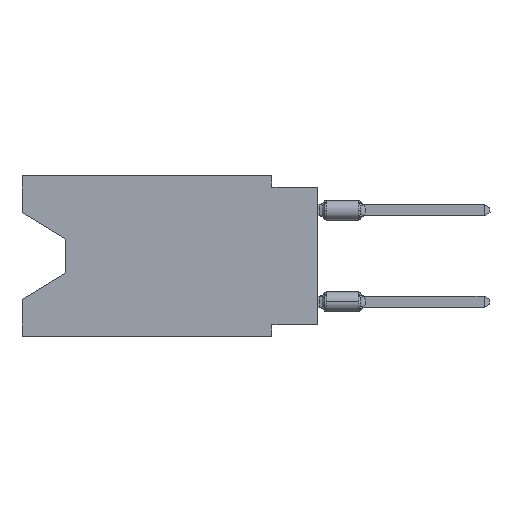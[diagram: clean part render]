
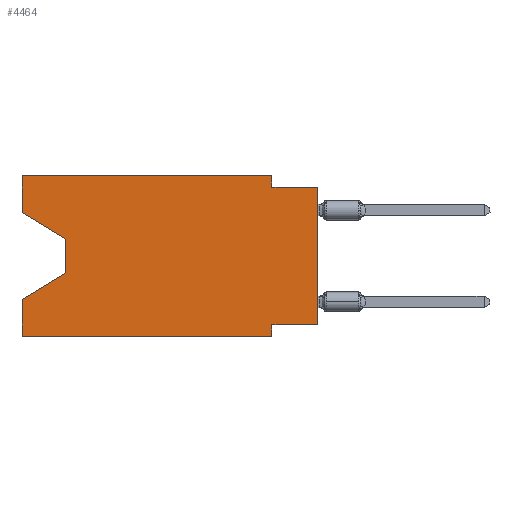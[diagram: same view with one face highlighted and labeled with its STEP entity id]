
A CAD part, left-side view. The second image highlights one B-rep face of the part: STEP entity #4464.
In plain terms, the highlighted planar face has unit normal (-1, 0, 0).
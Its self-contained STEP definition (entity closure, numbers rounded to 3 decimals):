
#127 = EDGE_CURVE ( 'NONE', #20466, #29470, #26719, .T. ) ;
#238 = DIRECTION ( 'NONE',  ( 0., 0., -1. ) ) ;
#277 = CARTESIAN_POINT ( 'NONE',  ( 0., 16.383, -2.038 ) ) ;
#307 = VERTEX_POINT ( 'NONE', #22963 ) ;
#825 = DIRECTION ( 'NONE',  ( 0., 0.855, -0.519 ) ) ;
#912 = VECTOR ( 'NONE', #4935, 1000. ) ;
#986 = CARTESIAN_POINT ( 'NONE',  ( 0., 13.97, -5.385 ) ) ;
#1016 = VERTEX_POINT ( 'NONE', #8411 ) ;
#1348 = VERTEX_POINT ( 'NONE', #986 ) ;
#1746 = EDGE_CURVE ( 'NONE', #307, #1348, #17062, .T. ) ;
#1863 = VECTOR ( 'NONE', #26538, 1000. ) ;
#1892 = DIRECTION ( 'NONE',  ( 0., -0.855, -0.519 ) ) ;
#2112 = CARTESIAN_POINT ( 'NONE',  ( 0., 0., -0.635 ) ) ;
#2147 = CARTESIAN_POINT ( 'NONE',  ( 0., 0., 0. ) ) ;
#2938 = VECTOR ( 'NONE', #26191, 1000. ) ;
#3699 = CARTESIAN_POINT ( 'NONE',  ( 0., 16.383, 0. ) ) ;
#3828 = VECTOR ( 'NONE', #28101, 1000. ) ;
#4464 = ADVANCED_FACE ( 'NONE', ( #6754 ), #16173, .F. ) ;
#4853 = LINE ( 'NONE', #12259, #29091 ) ;
#4935 = DIRECTION ( 'NONE',  ( 0., 1., 0. ) ) ;
#5178 = EDGE_CURVE ( 'NONE', #7450, #18401, #17626, .T. ) ;
#5221 = VERTEX_POINT ( 'NONE', #19931 ) ;
#5385 = VECTOR ( 'NONE', #11544, 1000. ) ;
#5508 = CARTESIAN_POINT ( 'NONE',  ( 0., 0., -8.255 ) ) ;
#6181 = CARTESIAN_POINT ( 'NONE',  ( 0., 2.54, -0.635 ) ) ;
#6455 = CARTESIAN_POINT ( 'NONE',  ( 0., 16.383, 0. ) ) ;
#6513 = CARTESIAN_POINT ( 'NONE',  ( 0., 16.383, -2.038 ) ) ;
#6754 = FACE_OUTER_BOUND ( 'NONE', #8732, .T. ) ;
#6927 = VERTEX_POINT ( 'NONE', #28974 ) ;
#7450 = VERTEX_POINT ( 'NONE', #6181 ) ;
#7916 = LINE ( 'NONE', #12678, #8224 ) ;
#8224 = VECTOR ( 'NONE', #825, 1000. ) ;
#8411 = CARTESIAN_POINT ( 'NONE',  ( 0., 2.54, -8.255 ) ) ;
#8651 = ORIENTED_EDGE ( 'NONE', *, *, #22971, .F. ) ;
#8732 = EDGE_LOOP ( 'NONE', ( #28680, #16036, #20191, #23287, #11457, #8651, #28444, #9402, #25509, #11028, #11565, #10864 ) ) ;
#9210 = DIRECTION ( 'NONE',  ( 1., 0., 0. ) ) ;
#9402 = ORIENTED_EDGE ( 'NONE', *, *, #22420, .T. ) ;
#9541 = LINE ( 'NONE', #28402, #912 ) ;
#9698 = CARTESIAN_POINT ( 'NONE',  ( 0., 16.383, 0. ) ) ;
#9869 = LINE ( 'NONE', #19272, #25025 ) ;
#10098 = DIRECTION ( 'NONE',  ( 0., 0., -1. ) ) ;
#10293 = VERTEX_POINT ( 'NONE', #5508 ) ;
#10674 = EDGE_CURVE ( 'NONE', #29470, #7450, #4853, .T. ) ;
#10826 = CARTESIAN_POINT ( 'NONE',  ( 0., 0., -0.635 ) ) ;
#10864 = ORIENTED_EDGE ( 'NONE', *, *, #19400, .F. ) ;
#11028 = ORIENTED_EDGE ( 'NONE', *, *, #10674, .F. ) ;
#11457 = ORIENTED_EDGE ( 'NONE', *, *, #25524, .T. ) ;
#11544 = DIRECTION ( 'NONE',  ( 0., 0., 1. ) ) ;
#11565 = ORIENTED_EDGE ( 'NONE', *, *, #127, .F. ) ;
#12259 = CARTESIAN_POINT ( 'NONE',  ( 0., 2.54, 0. ) ) ;
#12345 = DIRECTION ( 'NONE',  ( 0., -1., 0. ) ) ;
#12559 = VECTOR ( 'NONE', #24381, 1000. ) ;
#12678 = CARTESIAN_POINT ( 'NONE',  ( 0., 13.97, -5.385 ) ) ;
#14000 = DIRECTION ( 'NONE',  ( 0., 0., -1. ) ) ;
#14806 = LINE ( 'NONE', #9698, #1863 ) ;
#16036 = ORIENTED_EDGE ( 'NONE', *, *, #1746, .T. ) ;
#16079 = CARTESIAN_POINT ( 'NONE',  ( 0., 16.383, 0. ) ) ;
#16173 = PLANE ( 'NONE',  #30068 ) ;
#16773 = CARTESIAN_POINT ( 'NONE',  ( 0., 16.383, -6.852 ) ) ;
#17062 = LINE ( 'NONE', #21830, #27928 ) ;
#17350 = EDGE_CURVE ( 'NONE', #19780, #307, #18078, .T. ) ;
#17626 = LINE ( 'NONE', #10826, #20673 ) ;
#18078 = LINE ( 'NONE', #6513, #28411 ) ;
#18401 = VERTEX_POINT ( 'NONE', #2112 ) ;
#19272 = CARTESIAN_POINT ( 'NONE',  ( 0., 16.383, -8.89 ) ) ;
#19332 = EDGE_CURVE ( 'NONE', #6927, #23030, #20391, .T. ) ;
#19400 = EDGE_CURVE ( 'NONE', #19780, #20466, #14806, .T. ) ;
#19473 = EDGE_CURVE ( 'NONE', #10293, #1016, #9541, .T. ) ;
#19780 = VERTEX_POINT ( 'NONE', #277 ) ;
#19931 = CARTESIAN_POINT ( 'NONE',  ( 0., 2.54, -8.89 ) ) ;
#20191 = ORIENTED_EDGE ( 'NONE', *, *, #27481, .T. ) ;
#20391 = LINE ( 'NONE', #27512, #3828 ) ;
#20466 = VERTEX_POINT ( 'NONE', #16079 ) ;
#20673 = VECTOR ( 'NONE', #29388, 1000. ) ;
#21830 = CARTESIAN_POINT ( 'NONE',  ( 0., 13.97, -3.505 ) ) ;
#22420 = EDGE_CURVE ( 'NONE', #10293, #18401, #22812, .T. ) ;
#22812 = LINE ( 'NONE', #2147, #5385 ) ;
#22963 = CARTESIAN_POINT ( 'NONE',  ( 0., 13.97, -3.505 ) ) ;
#22971 = EDGE_CURVE ( 'NONE', #1016, #5221, #28690, .T. ) ;
#23030 = VERTEX_POINT ( 'NONE', #16773 ) ;
#23287 = ORIENTED_EDGE ( 'NONE', *, *, #19332, .F. ) ;
#24381 = DIRECTION ( 'NONE',  ( 0., -1., 0. ) ) ;
#25025 = VECTOR ( 'NONE', #12345, 1000. ) ;
#25509 = ORIENTED_EDGE ( 'NONE', *, *, #5178, .F. ) ;
#25524 = EDGE_CURVE ( 'NONE', #6927, #5221, #9869, .T. ) ;
#25539 = CARTESIAN_POINT ( 'NONE',  ( 0., 2.54, 0. ) ) ;
#26191 = DIRECTION ( 'NONE',  ( 0., 0., -1. ) ) ;
#26538 = DIRECTION ( 'NONE',  ( 0., 0., 1. ) ) ;
#26719 = LINE ( 'NONE', #3699, #12559 ) ;
#27481 = EDGE_CURVE ( 'NONE', #1348, #23030, #7916, .T. ) ;
#27512 = CARTESIAN_POINT ( 'NONE',  ( 0., 16.383, 0. ) ) ;
#27928 = VECTOR ( 'NONE', #10098, 1000. ) ;
#28101 = DIRECTION ( 'NONE',  ( 0., 0., 1. ) ) ;
#28402 = CARTESIAN_POINT ( 'NONE',  ( 0., 0., -8.255 ) ) ;
#28411 = VECTOR ( 'NONE', #1892, 1000. ) ;
#28444 = ORIENTED_EDGE ( 'NONE', *, *, #19473, .F. ) ;
#28522 = CARTESIAN_POINT ( 'NONE',  ( 0., 2.54, -8.89 ) ) ;
#28680 = ORIENTED_EDGE ( 'NONE', *, *, #17350, .T. ) ;
#28690 = LINE ( 'NONE', #28522, #2938 ) ;
#28974 = CARTESIAN_POINT ( 'NONE',  ( 0., 16.383, -8.89 ) ) ;
#29091 = VECTOR ( 'NONE', #238, 1000. ) ;
#29388 = DIRECTION ( 'NONE',  ( 0., -1., 0. ) ) ;
#29470 = VERTEX_POINT ( 'NONE', #25539 ) ;
#30068 = AXIS2_PLACEMENT_3D ( 'NONE', #6455, #9210, #14000 ) ;
